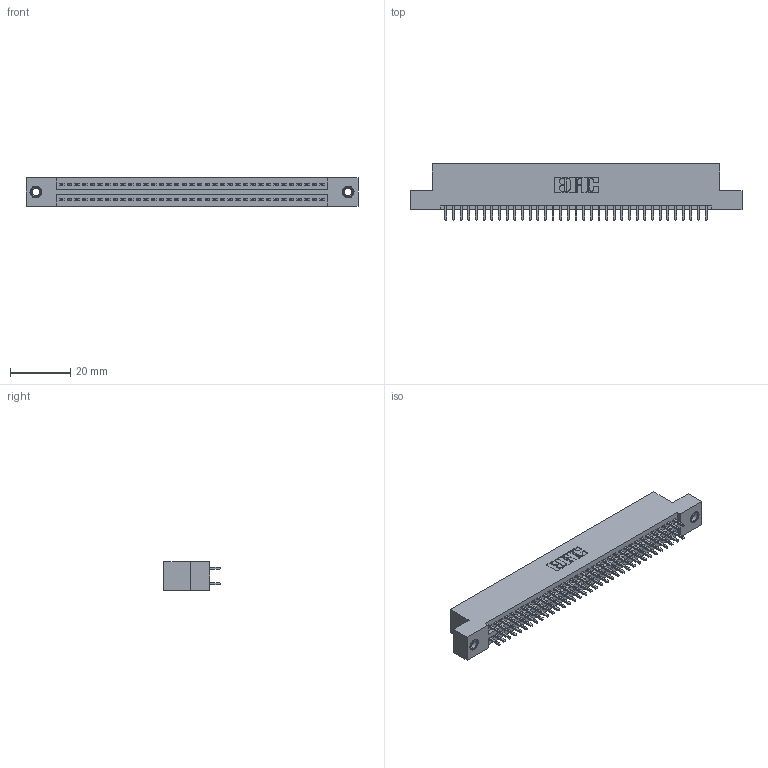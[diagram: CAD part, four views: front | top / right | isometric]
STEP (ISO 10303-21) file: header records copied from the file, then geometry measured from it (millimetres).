
FILE_DESCRIPTION (( 'STEP AP203' ), '1' );
FILE_NAME ('395-070-521-207.STEP', '2018-11-26T14:37:37', ( '' ), ( '' ), 'SwSTEP 2.0', 'SolidWorks 2016', '' );
FILE_SCHEMA (( 'CONFIG_CONTROL_DESIGN' ));
Length unit declared in the file: inch
Products named in the file (4): 345-292-001_345-293-121; 345-250-001_345-250-005-103; 395-070-521-207; 345 Part_Flush Mounting Lugs - 0.156 Dia-TI
Assembly tree (73 placements, depth 2):
  395-070-521-207
    345 Part_Flush Mounting Lugs - 0.156 Dia-TI
    345-292-001_345-293-121  x70
    345-250-001_345-250-005-103  x2
Bounding box: 110.11 x 18.72 x 9.4 mm (x, y, z)
Volume: 10589 mm3; surface area: 15358.7 mm2
Topology: 73 solids, 73 shells, 3686 faces, 10907 edges, 7170 vertices
Faces by surface type: plane 2422, cylinder 1248, cone 12, torus 4
Entity records: 29608 total; most frequent: CARTESIAN_POINT 4951, ORIENTED_EDGE 4878, DIRECTION 4401, EDGE_CURVE 2439, LINE 2147, VECTOR 2147, VERTEX_POINT 1620, AXIS2_PLACEMENT_3D 1127
